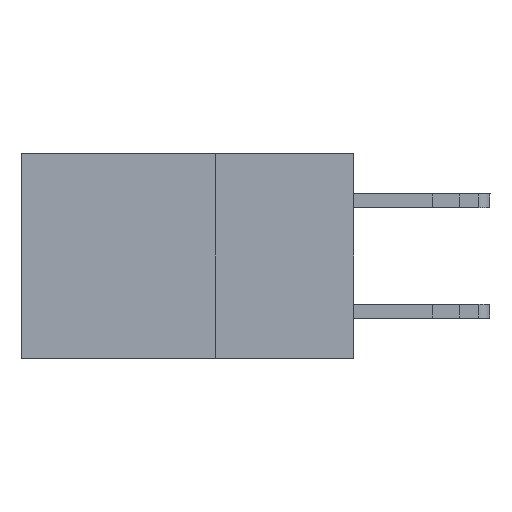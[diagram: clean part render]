
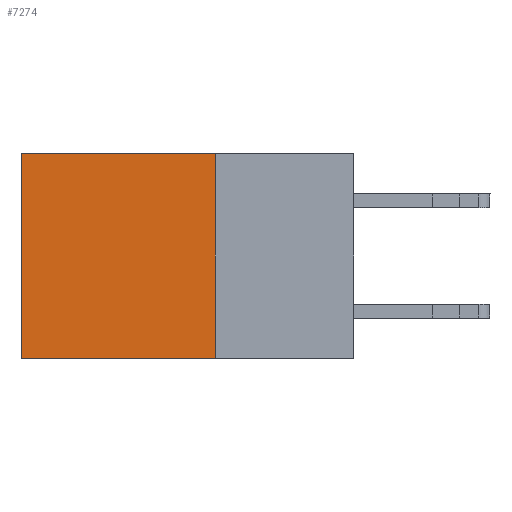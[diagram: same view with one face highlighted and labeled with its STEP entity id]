
A CAD part, left-side view. The second image highlights one B-rep face of the part: STEP entity #7274.
In plain terms, the highlighted planar face has unit normal (-1, 0, 0).
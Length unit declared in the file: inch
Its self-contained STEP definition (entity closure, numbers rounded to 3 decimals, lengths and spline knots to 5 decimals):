
#793 = VECTOR ( 'NONE', #1789, 39.37008 ) ;
#1035 = EDGE_LOOP ( 'NONE', ( #11851, #10446, #6518, #10832 ) ) ;
#1585 = LINE ( 'NONE', #14072, #18027 ) ;
#1787 = CARTESIAN_POINT ( 'NONE',  ( 0.2875, 0.25, 0. ) ) ;
#1789 = DIRECTION ( 'NONE',  ( 0., 0., -1. ) ) ;
#2643 = CARTESIAN_POINT ( 'NONE',  ( 0.2875, 0.25, -0.37 ) ) ;
#2853 = CARTESIAN_POINT ( 'NONE',  ( 0.2875, 0.25, 0. ) ) ;
#3233 = VERTEX_POINT ( 'NONE', #11042 ) ;
#3457 = AXIS2_PLACEMENT_3D ( 'NONE', #1787, #7856, #12015 ) ;
#4469 = EDGE_CURVE ( 'NONE', #4817, #10538, #1585, .T. ) ;
#4817 = VERTEX_POINT ( 'NONE', #2643 ) ;
#5128 = FACE_OUTER_BOUND ( 'NONE', #1035, .T. ) ;
#5271 = VECTOR ( 'NONE', #12699, 39.37008 ) ;
#6518 = ORIENTED_EDGE ( 'NONE', *, *, #12398, .F. ) ;
#7081 = DIRECTION ( 'NONE',  ( 0., 1., 0. ) ) ;
#7133 = DIRECTION ( 'NONE',  ( 0., 0., -1. ) ) ;
#7274 = ADVANCED_FACE ( 'NONE', ( #5128 ), #16713, .F. ) ;
#7856 = DIRECTION ( 'NONE',  ( 1., 0., 0. ) ) ;
#9372 = EDGE_CURVE ( 'NONE', #3233, #18607, #10557, .T. ) ;
#10446 = ORIENTED_EDGE ( 'NONE', *, *, #4469, .F. ) ;
#10538 = VERTEX_POINT ( 'NONE', #15935 ) ;
#10557 = LINE ( 'NONE', #15662, #5271 ) ;
#10832 = ORIENTED_EDGE ( 'NONE', *, *, #9372, .T. ) ;
#11042 = CARTESIAN_POINT ( 'NONE',  ( 0.2875, 0.25, 0. ) ) ;
#11851 = ORIENTED_EDGE ( 'NONE', *, *, #14269, .T. ) ;
#12015 = DIRECTION ( 'NONE',  ( 0., 0., -1. ) ) ;
#12141 = CARTESIAN_POINT ( 'NONE',  ( 0.2875, 0.6, 0. ) ) ;
#12301 = LINE ( 'NONE', #12141, #793 ) ;
#12398 = EDGE_CURVE ( 'NONE', #3233, #4817, #14442, .T. ) ;
#12699 = DIRECTION ( 'NONE',  ( 0., 1., 0. ) ) ;
#14072 = CARTESIAN_POINT ( 'NONE',  ( 0.2875, 0.25, -0.37 ) ) ;
#14269 = EDGE_CURVE ( 'NONE', #18607, #10538, #12301, .T. ) ;
#14442 = LINE ( 'NONE', #2853, #19029 ) ;
#15662 = CARTESIAN_POINT ( 'NONE',  ( 0.2875, 0.25, 0. ) ) ;
#15935 = CARTESIAN_POINT ( 'NONE',  ( 0.2875, 0.6, -0.37 ) ) ;
#16713 = PLANE ( 'NONE',  #3457 ) ;
#16780 = CARTESIAN_POINT ( 'NONE',  ( 0.2875, 0.6, 0. ) ) ;
#18027 = VECTOR ( 'NONE', #7081, 39.37008 ) ;
#18607 = VERTEX_POINT ( 'NONE', #16780 ) ;
#19029 = VECTOR ( 'NONE', #7133, 39.37008 ) ;
